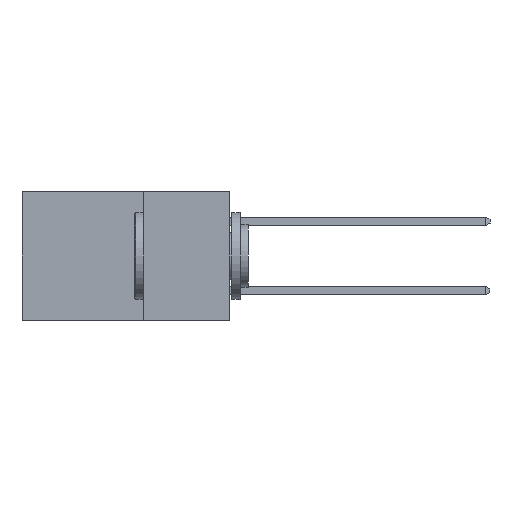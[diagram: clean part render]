
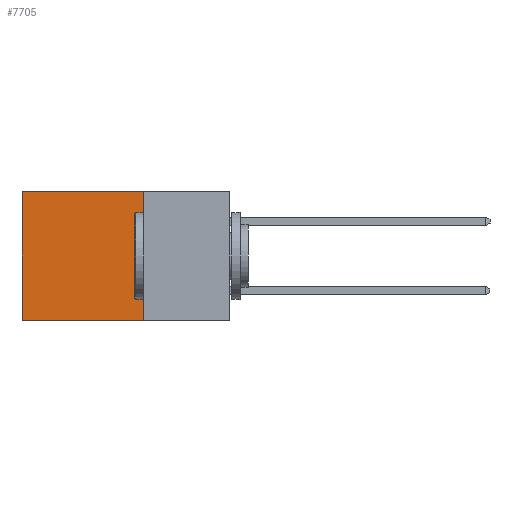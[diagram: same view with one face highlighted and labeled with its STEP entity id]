
A CAD part, left-side view. The second image highlights one B-rep face of the part: STEP entity #7705.
In plain terms, the highlighted planar face has unit normal (-1, 0, 0).
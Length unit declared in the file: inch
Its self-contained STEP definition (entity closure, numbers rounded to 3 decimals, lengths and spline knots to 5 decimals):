
#446 = DIRECTION ( 'NONE',  ( 0., 0., -1. ) ) ;
#509 = EDGE_LOOP ( 'NONE', ( #11415, #8768, #4252, #10092 ) ) ;
#952 = VERTEX_POINT ( 'NONE', #7731 ) ;
#1220 = CARTESIAN_POINT ( 'NONE',  ( 0.298, 0.6, -0.37 ) ) ;
#1246 = CARTESIAN_POINT ( 'NONE',  ( 0.298, 0.25, 0. ) ) ;
#1396 = DIRECTION ( 'NONE',  ( 0., 0., -1. ) ) ;
#1797 = FACE_OUTER_BOUND ( 'NONE', #509, .T. ) ;
#1963 = VECTOR ( 'NONE', #7469, 39.37008 ) ;
#3984 = PLANE ( 'NONE',  #5832 ) ;
#4212 = VECTOR ( 'NONE', #10831, 39.37008 ) ;
#4252 = ORIENTED_EDGE ( 'NONE', *, *, #8101, .F. ) ;
#4441 = CARTESIAN_POINT ( 'NONE',  ( 0.298, 0.25, -0.37 ) ) ;
#5013 = DIRECTION ( 'NONE',  ( 0., 0., -1. ) ) ;
#5041 = DIRECTION ( 'NONE',  ( 1., 0., 0. ) ) ;
#5057 = CARTESIAN_POINT ( 'NONE',  ( 0.298, 0.25, 0. ) ) ;
#5203 = VERTEX_POINT ( 'NONE', #1220 ) ;
#5315 = VECTOR ( 'NONE', #446, 39.37008 ) ;
#5706 = CARTESIAN_POINT ( 'NONE',  ( 0.298, 0.6, 0. ) ) ;
#5832 = AXIS2_PLACEMENT_3D ( 'NONE', #5057, #5041, #5013 ) ;
#6166 = CARTESIAN_POINT ( 'NONE',  ( 0.298, 0.25, -0.37 ) ) ;
#6411 = CARTESIAN_POINT ( 'NONE',  ( 0.298, 0.25, 0. ) ) ;
#7029 = LINE ( 'NONE', #4441, #4212 ) ;
#7469 = DIRECTION ( 'NONE',  ( 0., 1., 0. ) ) ;
#7705 = ADVANCED_FACE ( 'NONE', ( #1797 ), #3984, .F. ) ;
#7731 = CARTESIAN_POINT ( 'NONE',  ( 0.298, 0.25, 0. ) ) ;
#8101 = EDGE_CURVE ( 'NONE', #952, #13679, #10973, .T. ) ;
#8768 = ORIENTED_EDGE ( 'NONE', *, *, #9902, .F. ) ;
#9902 = EDGE_CURVE ( 'NONE', #13679, #5203, #7029, .T. ) ;
#10092 = ORIENTED_EDGE ( 'NONE', *, *, #11285, .T. ) ;
#10831 = DIRECTION ( 'NONE',  ( 0., 1., 0. ) ) ;
#10973 = LINE ( 'NONE', #1246, #5315 ) ;
#11133 = LINE ( 'NONE', #5706, #13576 ) ;
#11285 = EDGE_CURVE ( 'NONE', #952, #12684, #12938, .T. ) ;
#11415 = ORIENTED_EDGE ( 'NONE', *, *, #12080, .T. ) ;
#11971 = CARTESIAN_POINT ( 'NONE',  ( 0.298, 0.6, 0. ) ) ;
#12080 = EDGE_CURVE ( 'NONE', #12684, #5203, #11133, .T. ) ;
#12684 = VERTEX_POINT ( 'NONE', #11971 ) ;
#12938 = LINE ( 'NONE', #6411, #1963 ) ;
#13576 = VECTOR ( 'NONE', #1396, 39.37008 ) ;
#13679 = VERTEX_POINT ( 'NONE', #6166 ) ;
